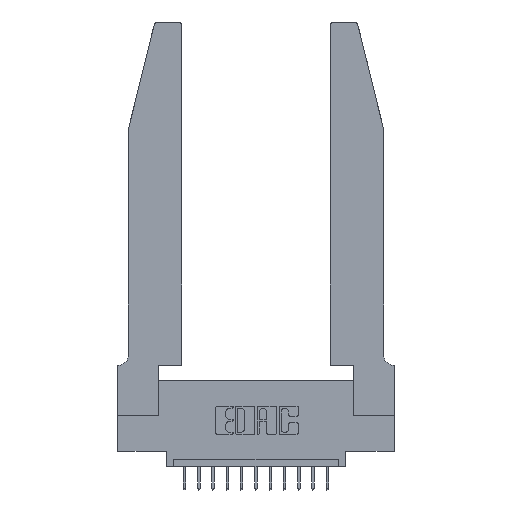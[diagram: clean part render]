
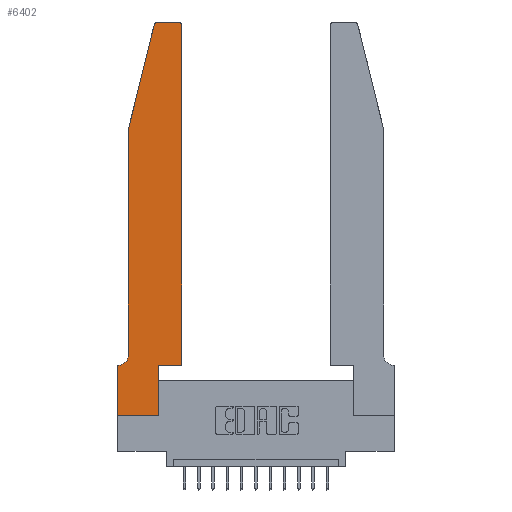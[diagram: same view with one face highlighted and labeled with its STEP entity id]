
A CAD part, top view. The second image highlights one B-rep face of the part: STEP entity #6402.
In plain terms, the highlighted planar face has unit normal (0, 0, 1).
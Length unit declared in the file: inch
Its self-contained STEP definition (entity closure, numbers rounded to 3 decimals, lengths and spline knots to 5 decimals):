
#3 = VERTEX_POINT ( 'NONE', #12838 ) ;
#287 = EDGE_CURVE ( 'NONE', #1702, #2407, #10400, .T. ) ;
#762 = PLANE ( 'NONE',  #7657 ) ;
#931 = VECTOR ( 'NONE', #11779, 39.37008 ) ;
#1300 = CARTESIAN_POINT ( 'NONE',  ( 0.0755, 0.42, 0.37 ) ) ;
#1550 = AXIS2_PLACEMENT_3D ( 'NONE', #15584, #12991, #6277 ) ;
#1655 = VERTEX_POINT ( 'NONE', #13931 ) ;
#1702 = VERTEX_POINT ( 'NONE', #12938 ) ;
#1824 = LINE ( 'NONE', #4571, #11726 ) ;
#1902 = VECTOR ( 'NONE', #13071, 39.37008 ) ;
#1922 = DIRECTION ( 'NONE',  ( -1., 0., 0. ) ) ;
#2407 = VERTEX_POINT ( 'NONE', #1300 ) ;
#2479 = EDGE_CURVE ( 'NONE', #1655, #6269, #7182, .T. ) ;
#2495 = ORIENTED_EDGE ( 'NONE', *, *, #5550, .T. ) ;
#2857 = EDGE_CURVE ( 'NONE', #3, #1702, #7165, .T. ) ;
#3117 = VECTOR ( 'NONE', #7600, 39.37008 ) ;
#3125 = CARTESIAN_POINT ( 'NONE',  ( 0.4505, 2.72, 0.37 ) ) ;
#3172 = DIRECTION ( 'NONE',  ( 0., 0., 1. ) ) ;
#3286 = CARTESIAN_POINT ( 'NONE',  ( 0.284, 2.72, 0.37 ) ) ;
#3659 = VECTOR ( 'NONE', #16729, 39.37008 ) ;
#3886 = DIRECTION ( 'NONE',  ( -0.239, -0.971, 0. ) ) ;
#4027 = EDGE_CURVE ( 'NONE', #15907, #9034, #8208, .T. ) ;
#4074 = EDGE_LOOP ( 'NONE', ( #2495, #8054, #6761, #15955, #10612, #11868, #6946, #12344, #8991, #12897, #7729, #13810 ) ) ;
#4352 = CARTESIAN_POINT ( 'NONE',  ( 0.284, 2.75, 0.37 ) ) ;
#4416 = LINE ( 'NONE', #4790, #931 ) ;
#4571 = CARTESIAN_POINT ( 'NONE',  ( 0.2605, 2.75, 0.37 ) ) ;
#4790 = CARTESIAN_POINT ( 'NONE',  ( 0.4505, 0.35, 0.37 ) ) ;
#4817 = CARTESIAN_POINT ( 'NONE',  ( 0.0755, 0.35, 0.37 ) ) ;
#4953 = EDGE_CURVE ( 'NONE', #5508, #3, #8571, .T. ) ;
#5251 = DIRECTION ( 'NONE',  ( 0., -1., 0. ) ) ;
#5338 = CARTESIAN_POINT ( 'NONE',  ( 0.4505, 0.35, 0.37 ) ) ;
#5349 = VERTEX_POINT ( 'NONE', #10636 ) ;
#5508 = VERTEX_POINT ( 'NONE', #4352 ) ;
#5550 = EDGE_CURVE ( 'NONE', #11740, #5508, #1824, .T. ) ;
#5953 = VECTOR ( 'NONE', #5251, 39.37008 ) ;
#6269 = VERTEX_POINT ( 'NONE', #12804 ) ;
#6277 = DIRECTION ( 'NONE',  ( 1., 0., 0. ) ) ;
#6312 = VERTEX_POINT ( 'NONE', #3125 ) ;
#6382 = EDGE_CURVE ( 'NONE', #7069, #5349, #15717, .T. ) ;
#6402 = ADVANCED_FACE ( 'NONE', ( #8529 ), #762, .T. ) ;
#6599 = AXIS2_PLACEMENT_3D ( 'NONE', #3286, #3172, #13974 ) ;
#6611 = LINE ( 'NONE', #7391, #9152 ) ;
#6761 = ORIENTED_EDGE ( 'NONE', *, *, #2857, .T. ) ;
#6825 = CARTESIAN_POINT ( 'NONE',  ( 0., 0., 0.37 ) ) ;
#6850 = EDGE_CURVE ( 'NONE', #6312, #11740, #13586, .T. ) ;
#6946 = ORIENTED_EDGE ( 'NONE', *, *, #9712, .T. ) ;
#7069 = VERTEX_POINT ( 'NONE', #16888 ) ;
#7165 = LINE ( 'NONE', #9225, #10533 ) ;
#7182 = LINE ( 'NONE', #7954, #1902 ) ;
#7391 = CARTESIAN_POINT ( 'NONE',  ( 0.2865, 0.35, 0.37 ) ) ;
#7469 = CIRCLE ( 'NONE', #12822, 0.07 ) ;
#7484 = DIRECTION ( 'NONE',  ( -1., 0., 0. ) ) ;
#7600 = DIRECTION ( 'NONE',  ( -1., 0., 0. ) ) ;
#7657 = AXIS2_PLACEMENT_3D ( 'NONE', #12787, #17147, #15803 ) ;
#7729 = ORIENTED_EDGE ( 'NONE', *, *, #9996, .T. ) ;
#7954 = CARTESIAN_POINT ( 'NONE',  ( 0., 0., 0.37 ) ) ;
#8054 = ORIENTED_EDGE ( 'NONE', *, *, #4953, .T. ) ;
#8179 = CARTESIAN_POINT ( 'NONE',  ( 0., 0.35, 0.37 ) ) ;
#8208 = LINE ( 'NONE', #4817, #3117 ) ;
#8529 = FACE_OUTER_BOUND ( 'NONE', #4074, .T. ) ;
#8571 = CIRCLE ( 'NONE', #6599, 0.03 ) ;
#8991 = ORIENTED_EDGE ( 'NONE', *, *, #9041, .T. ) ;
#9034 = VERTEX_POINT ( 'NONE', #8179 ) ;
#9041 = EDGE_CURVE ( 'NONE', #6269, #7069, #6611, .T. ) ;
#9152 = VECTOR ( 'NONE', #13153, 39.37008 ) ;
#9225 = CARTESIAN_POINT ( 'NONE',  ( 0.0755, 2., 0.37 ) ) ;
#9712 = EDGE_CURVE ( 'NONE', #9034, #1655, #16496, .T. ) ;
#9996 = EDGE_CURVE ( 'NONE', #5349, #6312, #4416, .T. ) ;
#10400 = LINE ( 'NONE', #13537, #5953 ) ;
#10533 = VECTOR ( 'NONE', #3886, 39.37008 ) ;
#10612 = ORIENTED_EDGE ( 'NONE', *, *, #16278, .T. ) ;
#10636 = CARTESIAN_POINT ( 'NONE',  ( 0.4505, 0.35, 0.37 ) ) ;
#11726 = VECTOR ( 'NONE', #1922, 39.37008 ) ;
#11740 = VERTEX_POINT ( 'NONE', #12033 ) ;
#11779 = DIRECTION ( 'NONE',  ( 0., 1., 0. ) ) ;
#11868 = ORIENTED_EDGE ( 'NONE', *, *, #4027, .T. ) ;
#12033 = CARTESIAN_POINT ( 'NONE',  ( 0.4205, 2.75, 0.37 ) ) ;
#12344 = ORIENTED_EDGE ( 'NONE', *, *, #2479, .T. ) ;
#12787 = CARTESIAN_POINT ( 'NONE',  ( 0., 0.35, 0.37 ) ) ;
#12804 = CARTESIAN_POINT ( 'NONE',  ( 0.2865, 0., 0.37 ) ) ;
#12822 = AXIS2_PLACEMENT_3D ( 'NONE', #14176, #16871, #7484 ) ;
#12838 = CARTESIAN_POINT ( 'NONE',  ( 0.25487, 2.72718, 0.37 ) ) ;
#12897 = ORIENTED_EDGE ( 'NONE', *, *, #6382, .T. ) ;
#12938 = CARTESIAN_POINT ( 'NONE',  ( 0.0755, 2., 0.37 ) ) ;
#12991 = DIRECTION ( 'NONE',  ( 0., 0., 1. ) ) ;
#13071 = DIRECTION ( 'NONE',  ( 1., 0., 0. ) ) ;
#13153 = DIRECTION ( 'NONE',  ( 0., 1., 0. ) ) ;
#13537 = CARTESIAN_POINT ( 'NONE',  ( 0.0755, 2., 0.37 ) ) ;
#13586 = CIRCLE ( 'NONE', #1550, 0.03 ) ;
#13810 = ORIENTED_EDGE ( 'NONE', *, *, #6850, .T. ) ;
#13931 = CARTESIAN_POINT ( 'NONE',  ( 0., 0., 0.37 ) ) ;
#13974 = DIRECTION ( 'NONE',  ( 1., 0., 0. ) ) ;
#14176 = CARTESIAN_POINT ( 'NONE',  ( 0.0055, 0.42, 0.37 ) ) ;
#15174 = DIRECTION ( 'NONE',  ( 0., -1., 0. ) ) ;
#15584 = CARTESIAN_POINT ( 'NONE',  ( 0.4205, 2.72, 0.37 ) ) ;
#15717 = LINE ( 'NONE', #5338, #3659 ) ;
#15803 = DIRECTION ( 'NONE',  ( 1., 0., 0. ) ) ;
#15907 = VERTEX_POINT ( 'NONE', #16208 ) ;
#15955 = ORIENTED_EDGE ( 'NONE', *, *, #287, .T. ) ;
#16208 = CARTESIAN_POINT ( 'NONE',  ( 0.0055, 0.35, 0.37 ) ) ;
#16278 = EDGE_CURVE ( 'NONE', #2407, #15907, #7469, .T. ) ;
#16496 = LINE ( 'NONE', #6825, #17369 ) ;
#16729 = DIRECTION ( 'NONE',  ( 1., 0., 0. ) ) ;
#16871 = DIRECTION ( 'NONE',  ( 0., 0., -1. ) ) ;
#16888 = CARTESIAN_POINT ( 'NONE',  ( 0.2865, 0.35, 0.37 ) ) ;
#17147 = DIRECTION ( 'NONE',  ( 0., 0., 1. ) ) ;
#17369 = VECTOR ( 'NONE', #15174, 39.37008 ) ;
